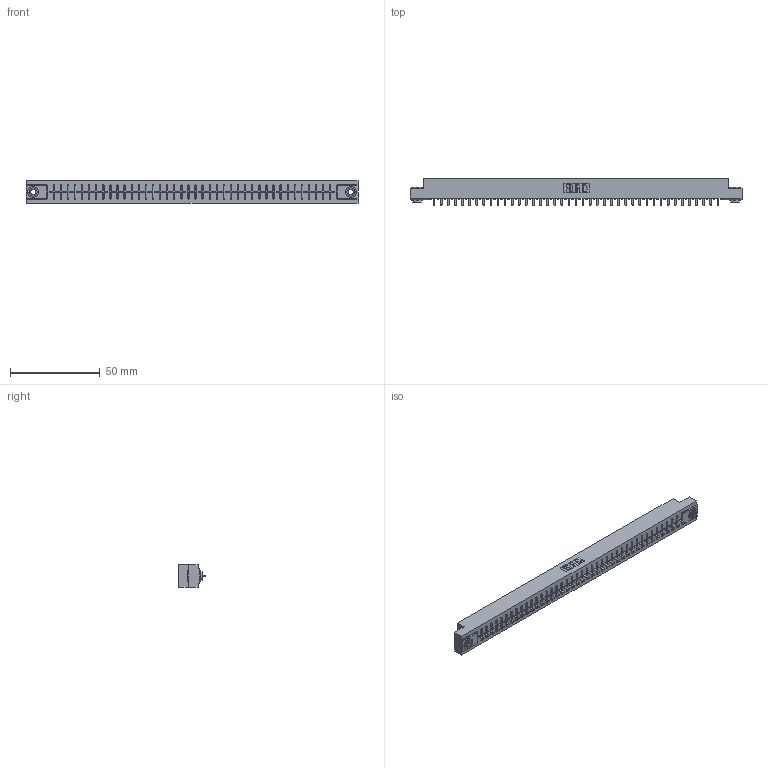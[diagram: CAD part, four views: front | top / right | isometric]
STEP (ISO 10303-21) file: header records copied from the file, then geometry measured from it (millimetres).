
FILE_DESCRIPTION (( 'STEP AP203' ), '1' );
FILE_NAME ('356-041-421-103.STEP', '2020-09-24T01:07:53', ( '' ), ( '' ), 'SwSTEP 2.0', 'SolidWorks 2020', '' );
FILE_SCHEMA (( 'CONFIG_CONTROL_DESIGN' ));
Length unit declared in the file: inch
Products named in the file (4): 356-041-421-103; 345-250-002_345-250-002-102; 306 Part_.156 Dia; 306-290-001_121
Assembly tree (44 placements, depth 2):
  356-041-421-103
    306 Part_.156 Dia
    306-290-001_121  x41
    345-250-002_345-250-002-102  x2
Bounding box: 185.47 x 14.88 x 12.7 mm (x, y, z)
Volume: 20450.5 mm3; surface area: 20938.3 mm2
Topology: 44 solids, 44 shells, 3038 faces, 8505 edges, 5446 vertices
Faces by surface type: plane 2019, cylinder 847, sphere 164, cone 8
Entity records: 39385 total; most frequent: CARTESIAN_POINT 6591, ORIENTED_EDGE 6526, DIRECTION 6513, EDGE_CURVE 3263, LINE 2545, VECTOR 2545, VERTEX_POINT 2062, AXIS2_PLACEMENT_3D 1984
